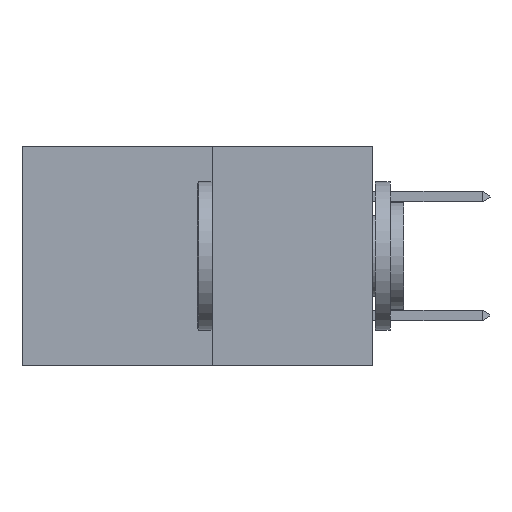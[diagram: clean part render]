
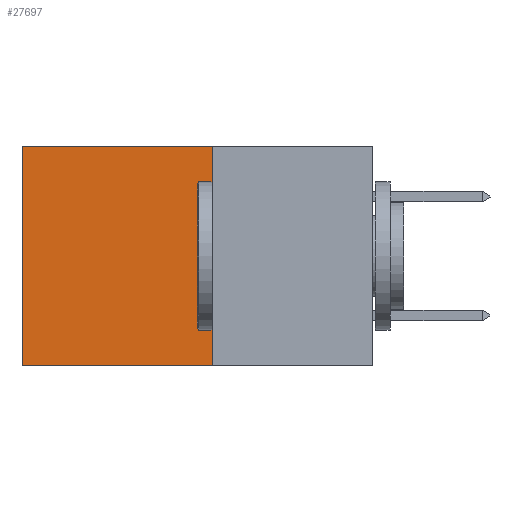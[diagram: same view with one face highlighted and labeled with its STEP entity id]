
A CAD part, left-side view. The second image highlights one B-rep face of the part: STEP entity #27697.
In plain terms, the highlighted planar face has unit normal (-1, 0, 0).
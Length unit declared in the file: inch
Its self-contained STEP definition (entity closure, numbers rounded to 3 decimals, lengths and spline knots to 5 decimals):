
#34 = CARTESIAN_POINT ( 'NONE',  ( 0.277, 0.59, 0. ) ) ;
#54 = DIRECTION ( 'NONE',  ( 0., 0., -1. ) ) ;
#840 = CARTESIAN_POINT ( 'NONE',  ( 0.277, 0.59, -0.37 ) ) ;
#2008 = CARTESIAN_POINT ( 'NONE',  ( 0.277, 0.27, 0. ) ) ;
#2724 = ORIENTED_EDGE ( 'NONE', *, *, #25571, .T. ) ;
#3040 = EDGE_LOOP ( 'NONE', ( #2724, #25343, #12635, #19459 ) ) ;
#3288 = VECTOR ( 'NONE', #14840, 39.37008 ) ;
#3599 = DIRECTION ( 'NONE',  ( 0., 0., -1. ) ) ;
#3610 = CARTESIAN_POINT ( 'NONE',  ( 0.277, 0.27, -0.37 ) ) ;
#3814 = EDGE_CURVE ( 'NONE', #18474, #11335, #3995, .T. ) ;
#3995 = LINE ( 'NONE', #3610, #3288 ) ;
#4587 = CARTESIAN_POINT ( 'NONE',  ( 0.277, 0.27, -0.37 ) ) ;
#5229 = DIRECTION ( 'NONE',  ( 0., 1., 0. ) ) ;
#6305 = FACE_OUTER_BOUND ( 'NONE', #3040, .T. ) ;
#6426 = EDGE_CURVE ( 'NONE', #18636, #16509, #23983, .T. ) ;
#7639 = EDGE_CURVE ( 'NONE', #18636, #18474, #10122, .T. ) ;
#10122 = LINE ( 'NONE', #4587, #15398 ) ;
#10330 = CARTESIAN_POINT ( 'NONE',  ( 0.277, 0.27, -0.37 ) ) ;
#10339 = LINE ( 'NONE', #840, #27618 ) ;
#11335 = VERTEX_POINT ( 'NONE', #22111 ) ;
#12495 = PLANE ( 'NONE',  #28575 ) ;
#12635 = ORIENTED_EDGE ( 'NONE', *, *, #7639, .F. ) ;
#14840 = DIRECTION ( 'NONE',  ( 0., 1., 0. ) ) ;
#15398 = VECTOR ( 'NONE', #54, 39.37008 ) ;
#16471 = CARTESIAN_POINT ( 'NONE',  ( 0.277, 0.27, 0. ) ) ;
#16509 = VERTEX_POINT ( 'NONE', #34 ) ;
#17108 = DIRECTION ( 'NONE',  ( 1., 0., 0. ) ) ;
#18474 = VERTEX_POINT ( 'NONE', #21726 ) ;
#18636 = VERTEX_POINT ( 'NONE', #2008 ) ;
#19459 = ORIENTED_EDGE ( 'NONE', *, *, #6426, .T. ) ;
#20970 = DIRECTION ( 'NONE',  ( 0., 0., -1. ) ) ;
#21726 = CARTESIAN_POINT ( 'NONE',  ( 0.277, 0.27, -0.37 ) ) ;
#22111 = CARTESIAN_POINT ( 'NONE',  ( 0.277, 0.59, -0.37 ) ) ;
#23246 = VECTOR ( 'NONE', #5229, 39.37008 ) ;
#23983 = LINE ( 'NONE', #16471, #23246 ) ;
#25343 = ORIENTED_EDGE ( 'NONE', *, *, #3814, .F. ) ;
#25571 = EDGE_CURVE ( 'NONE', #16509, #11335, #10339, .T. ) ;
#27618 = VECTOR ( 'NONE', #20970, 39.37008 ) ;
#27697 = ADVANCED_FACE ( 'NONE', ( #6305 ), #12495, .F. ) ;
#28575 = AXIS2_PLACEMENT_3D ( 'NONE', #10330, #17108, #3599 ) ;
